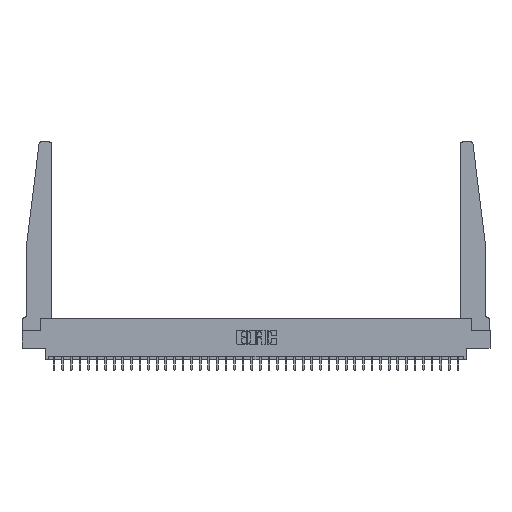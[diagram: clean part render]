
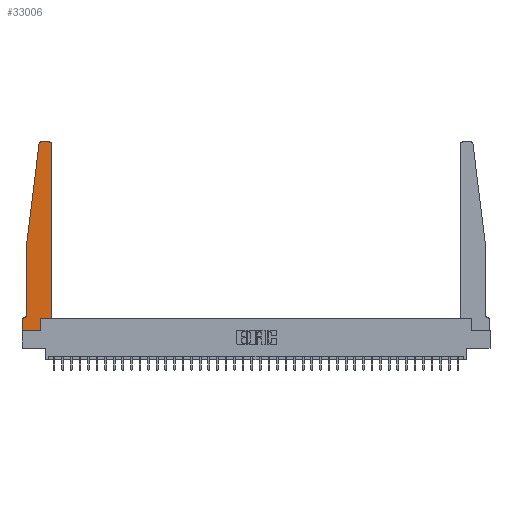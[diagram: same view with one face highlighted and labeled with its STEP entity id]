
A CAD part, top view. The second image highlights one B-rep face of the part: STEP entity #33006.
In plain terms, the highlighted planar face has unit normal (0, 0, 1).
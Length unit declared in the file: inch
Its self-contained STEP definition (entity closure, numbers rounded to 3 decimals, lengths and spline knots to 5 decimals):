
#68 = EDGE_CURVE ( 'NONE', #33922, #11589, #24877, .T. ) ;
#430 = ORIENTED_EDGE ( 'NONE', *, *, #27385, .T. ) ;
#506 = DIRECTION ( 'NONE',  ( 1., 0., 0. ) ) ;
#617 = AXIS2_PLACEMENT_3D ( 'NONE', #33381, #17181, #506 ) ;
#708 = EDGE_CURVE ( 'NONE', #23298, #7046, #14166, .T. ) ;
#721 = EDGE_CURVE ( 'NONE', #11589, #18003, #5896, .T. ) ;
#752 = VERTEX_POINT ( 'NONE', #21934 ) ;
#1786 = DIRECTION ( 'NONE',  ( -1., 0., 0. ) ) ;
#2325 = EDGE_CURVE ( 'NONE', #6944, #15256, #22162, .T. ) ;
#2584 = ORIENTED_EDGE ( 'NONE', *, *, #31193, .T. ) ;
#3123 = DIRECTION ( 'NONE',  ( 0., 0., -1. ) ) ;
#3767 = VECTOR ( 'NONE', #11168, 39.37008 ) ;
#3887 = VERTEX_POINT ( 'NONE', #4178 ) ;
#4066 = EDGE_CURVE ( 'NONE', #15256, #752, #29365, .T. ) ;
#4178 = CARTESIAN_POINT ( 'NONE',  ( 0.015, 0.1875, 0.37 ) ) ;
#4244 = CARTESIAN_POINT ( 'NONE',  ( 0.065, 1.25, 0.37 ) ) ;
#4607 = EDGE_LOOP ( 'NONE', ( #15680, #12077, #2584, #5541, #19881, #430, #6546, #12612, #21490, #34429, #10390, #13168 ) ) ;
#4908 = CARTESIAN_POINT ( 'NONE',  ( 0., 0.1875, 0.37 ) ) ;
#5012 = LINE ( 'NONE', #21861, #26084 ) ;
#5126 = VECTOR ( 'NONE', #20768, 39.37008 ) ;
#5540 = LINE ( 'NONE', #17858, #26598 ) ;
#5541 = ORIENTED_EDGE ( 'NONE', *, *, #29730, .T. ) ;
#5896 = LINE ( 'NONE', #21804, #19730 ) ;
#5949 = AXIS2_PLACEMENT_3D ( 'NONE', #19703, #3123, #22441 ) ;
#6456 = VECTOR ( 'NONE', #31283, 39.37008 ) ;
#6546 = ORIENTED_EDGE ( 'NONE', *, *, #708, .T. ) ;
#6615 = FACE_OUTER_BOUND ( 'NONE', #4607, .T. ) ;
#6944 = VERTEX_POINT ( 'NONE', #25554 ) ;
#6945 = CARTESIAN_POINT ( 'NONE',  ( 0., 0., 0.37 ) ) ;
#7046 = VERTEX_POINT ( 'NONE', #6945 ) ;
#7745 = VERTEX_POINT ( 'NONE', #22312 ) ;
#7964 = DIRECTION ( 'NONE',  ( 0., -1., 0. ) ) ;
#8351 = AXIS2_PLACEMENT_3D ( 'NONE', #11516, #30714, #14421 ) ;
#10390 = ORIENTED_EDGE ( 'NONE', *, *, #28391, .T. ) ;
#11039 = CARTESIAN_POINT ( 'NONE',  ( 0.065, 1.25, 0.37 ) ) ;
#11168 = DIRECTION ( 'NONE',  ( 0., 1., 0. ) ) ;
#11516 = CARTESIAN_POINT ( 'NONE',  ( 0., 0.1875, 0.37 ) ) ;
#11589 = VERTEX_POINT ( 'NONE', #22675 ) ;
#12077 = ORIENTED_EDGE ( 'NONE', *, *, #4066, .T. ) ;
#12210 = CARTESIAN_POINT ( 'NONE',  ( 0.425, 0.18, 0.37 ) ) ;
#12398 = CIRCLE ( 'NONE', #5949, 0.05 ) ;
#12612 = ORIENTED_EDGE ( 'NONE', *, *, #23069, .T. ) ;
#13144 = DIRECTION ( 'NONE',  ( 0., 0., 1. ) ) ;
#13168 = ORIENTED_EDGE ( 'NONE', *, *, #22614, .T. ) ;
#13398 = VERTEX_POINT ( 'NONE', #33185 ) ;
#14166 = LINE ( 'NONE', #16328, #27813 ) ;
#14421 = DIRECTION ( 'NONE',  ( 1., 0., 0. ) ) ;
#15256 = VERTEX_POINT ( 'NONE', #18932 ) ;
#15680 = ORIENTED_EDGE ( 'NONE', *, *, #2325, .T. ) ;
#16328 = CARTESIAN_POINT ( 'NONE',  ( 0., 0., 0.37 ) ) ;
#16516 = LINE ( 'NONE', #18299, #28434 ) ;
#17181 = DIRECTION ( 'NONE',  ( 0., 0., 1. ) ) ;
#17858 = CARTESIAN_POINT ( 'NONE',  ( 0., 0., 0.37 ) ) ;
#18003 = VERTEX_POINT ( 'NONE', #29351 ) ;
#18268 = EDGE_CURVE ( 'NONE', #13398, #3887, #12398, .T. ) ;
#18299 = CARTESIAN_POINT ( 'NONE',  ( 0.065, 0.1875, 0.37 ) ) ;
#18541 = CIRCLE ( 'NONE', #617, 0.03 ) ;
#18932 = CARTESIAN_POINT ( 'NONE',  ( 0.27653, 2.75, 0.37 ) ) ;
#19703 = CARTESIAN_POINT ( 'NONE',  ( 0.015, 0.2375, 0.37 ) ) ;
#19730 = VECTOR ( 'NONE', #24553, 39.37008 ) ;
#19881 = ORIENTED_EDGE ( 'NONE', *, *, #18268, .T. ) ;
#20272 = LINE ( 'NONE', #12210, #6456 ) ;
#20768 = DIRECTION ( 'NONE',  ( 0., -1., 0. ) ) ;
#21490 = ORIENTED_EDGE ( 'NONE', *, *, #68, .T. ) ;
#21804 = CARTESIAN_POINT ( 'NONE',  ( 0.425, 0.18, 0.37 ) ) ;
#21861 = CARTESIAN_POINT ( 'NONE',  ( 0.065, 1.25, 0.37 ) ) ;
#21934 = CARTESIAN_POINT ( 'NONE',  ( 0.24675, 2.72367, 0.37 ) ) ;
#22162 = LINE ( 'NONE', #33904, #28534 ) ;
#22312 = CARTESIAN_POINT ( 'NONE',  ( 0.425, 2.72, 0.37 ) ) ;
#22441 = DIRECTION ( 'NONE',  ( -1., 0., 0. ) ) ;
#22614 = EDGE_CURVE ( 'NONE', #7745, #6944, #18541, .T. ) ;
#22675 = CARTESIAN_POINT ( 'NONE',  ( 0.2605, 0.18, 0.37 ) ) ;
#23069 = EDGE_CURVE ( 'NONE', #7046, #33922, #5540, .T. ) ;
#23298 = VERTEX_POINT ( 'NONE', #4908 ) ;
#23681 = CARTESIAN_POINT ( 'NONE',  ( 0.2605, 0., 0.37 ) ) ;
#24553 = DIRECTION ( 'NONE',  ( 1., 0., 0. ) ) ;
#24877 = LINE ( 'NONE', #30267, #3767 ) ;
#25554 = CARTESIAN_POINT ( 'NONE',  ( 0.395, 2.75, 0.37 ) ) ;
#26084 = VECTOR ( 'NONE', #35396, 39.37008 ) ;
#26598 = VECTOR ( 'NONE', #34060, 39.37008 ) ;
#27282 = AXIS2_PLACEMENT_3D ( 'NONE', #29488, #13144, #32172 ) ;
#27385 = EDGE_CURVE ( 'NONE', #3887, #23298, #16516, .T. ) ;
#27627 = VERTEX_POINT ( 'NONE', #11039 ) ;
#27813 = VECTOR ( 'NONE', #7964, 39.37008 ) ;
#28014 = PLANE ( 'NONE',  #8351 ) ;
#28391 = EDGE_CURVE ( 'NONE', #18003, #7745, #20272, .T. ) ;
#28434 = VECTOR ( 'NONE', #1786, 39.37008 ) ;
#28534 = VECTOR ( 'NONE', #31212, 39.37008 ) ;
#29351 = CARTESIAN_POINT ( 'NONE',  ( 0.425, 0.18, 0.37 ) ) ;
#29365 = CIRCLE ( 'NONE', #27282, 0.03 ) ;
#29488 = CARTESIAN_POINT ( 'NONE',  ( 0.27653, 2.72, 0.37 ) ) ;
#29730 = EDGE_CURVE ( 'NONE', #27627, #13398, #35007, .T. ) ;
#30267 = CARTESIAN_POINT ( 'NONE',  ( 0.2605, 0.18, 0.37 ) ) ;
#30714 = DIRECTION ( 'NONE',  ( 0., 0., 1. ) ) ;
#31193 = EDGE_CURVE ( 'NONE', #752, #27627, #5012, .T. ) ;
#31212 = DIRECTION ( 'NONE',  ( -1., 0., 0. ) ) ;
#31283 = DIRECTION ( 'NONE',  ( 0., 1., 0. ) ) ;
#32172 = DIRECTION ( 'NONE',  ( 1., 0., 0. ) ) ;
#33006 = ADVANCED_FACE ( 'NONE', ( #6615 ), #28014, .T. ) ;
#33185 = CARTESIAN_POINT ( 'NONE',  ( 0.065, 0.2375, 0.37 ) ) ;
#33381 = CARTESIAN_POINT ( 'NONE',  ( 0.395, 2.72, 0.37 ) ) ;
#33904 = CARTESIAN_POINT ( 'NONE',  ( 0.25, 2.75, 0.37 ) ) ;
#33922 = VERTEX_POINT ( 'NONE', #23681 ) ;
#34060 = DIRECTION ( 'NONE',  ( 1., 0., 0. ) ) ;
#34429 = ORIENTED_EDGE ( 'NONE', *, *, #721, .T. ) ;
#35007 = LINE ( 'NONE', #4244, #5126 ) ;
#35396 = DIRECTION ( 'NONE',  ( -0.122, -0.992, 0. ) ) ;
